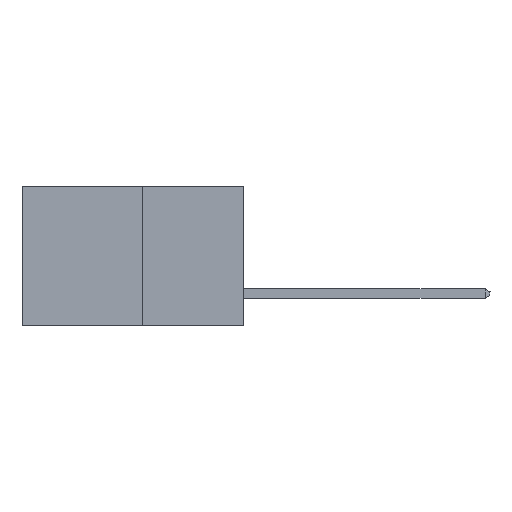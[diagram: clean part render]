
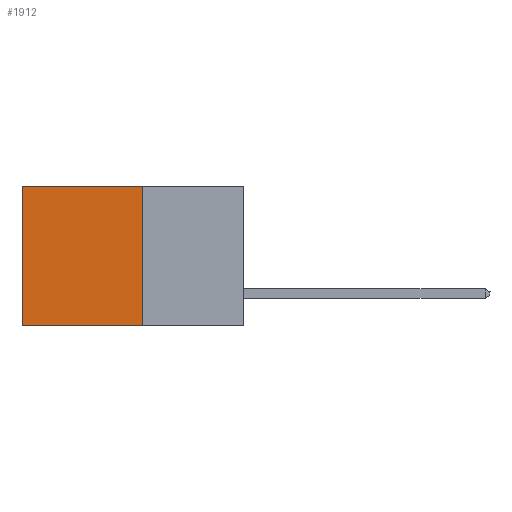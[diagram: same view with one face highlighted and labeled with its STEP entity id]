
A CAD part, left-side view. The second image highlights one B-rep face of the part: STEP entity #1912.
In plain terms, the highlighted planar face has unit normal (-1, 0, 0).
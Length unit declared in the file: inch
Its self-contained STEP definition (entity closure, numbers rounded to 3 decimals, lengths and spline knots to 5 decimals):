
#285 = EDGE_CURVE ( 'NONE', #6637, #10688, #9355, .T. ) ;
#1652 = CARTESIAN_POINT ( 'NONE',  ( 0.277, 0.27, -0.37 ) ) ;
#1794 = DIRECTION ( 'NONE',  ( 0., 0., -1. ) ) ;
#1912 = ADVANCED_FACE ( 'NONE', ( #9507 ), #6419, .F. ) ;
#2110 = CARTESIAN_POINT ( 'NONE',  ( 0.277, 0.27, -0.37 ) ) ;
#2352 = CARTESIAN_POINT ( 'NONE',  ( 0.277, 0.59, -0.37 ) ) ;
#2558 = DIRECTION ( 'NONE',  ( 0., 0., -1. ) ) ;
#3580 = ORIENTED_EDGE ( 'NONE', *, *, #6530, .T. ) ;
#3706 = CARTESIAN_POINT ( 'NONE',  ( 0.277, 0.27, 0. ) ) ;
#3796 = ORIENTED_EDGE ( 'NONE', *, *, #285, .F. ) ;
#3920 = ORIENTED_EDGE ( 'NONE', *, *, #5425, .F. ) ;
#4307 = ORIENTED_EDGE ( 'NONE', *, *, #9926, .T. ) ;
#4753 = DIRECTION ( 'NONE',  ( 0., 1., 0. ) ) ;
#5056 = AXIS2_PLACEMENT_3D ( 'NONE', #6396, #5975, #5937 ) ;
#5283 = VECTOR ( 'NONE', #4753, 39.37008 ) ;
#5425 = EDGE_CURVE ( 'NONE', #9113, #6637, #10570, .T. ) ;
#5875 = CARTESIAN_POINT ( 'NONE',  ( 0.277, 0.27, -0.37 ) ) ;
#5937 = DIRECTION ( 'NONE',  ( 0., 0., -1. ) ) ;
#5975 = DIRECTION ( 'NONE',  ( 1., 0., 0. ) ) ;
#6396 = CARTESIAN_POINT ( 'NONE',  ( 0.277, 0.27, -0.37 ) ) ;
#6419 = PLANE ( 'NONE',  #5056 ) ;
#6530 = EDGE_CURVE ( 'NONE', #11712, #10688, #10371, .T. ) ;
#6637 = VERTEX_POINT ( 'NONE', #1652 ) ;
#6646 = VECTOR ( 'NONE', #9625, 39.37008 ) ;
#7400 = CARTESIAN_POINT ( 'NONE',  ( 0.277, 0.27, 0. ) ) ;
#8408 = LINE ( 'NONE', #3706, #5283 ) ;
#9113 = VERTEX_POINT ( 'NONE', #7400 ) ;
#9355 = LINE ( 'NONE', #5875, #6646 ) ;
#9507 = FACE_OUTER_BOUND ( 'NONE', #9628, .T. ) ;
#9625 = DIRECTION ( 'NONE',  ( 0., 1., 0. ) ) ;
#9628 = EDGE_LOOP ( 'NONE', ( #3580, #3796, #3920, #4307 ) ) ;
#9806 = CARTESIAN_POINT ( 'NONE',  ( 0.277, 0.59, -0.37 ) ) ;
#9926 = EDGE_CURVE ( 'NONE', #9113, #11712, #8408, .T. ) ;
#10077 = VECTOR ( 'NONE', #2558, 39.37008 ) ;
#10371 = LINE ( 'NONE', #9806, #10077 ) ;
#10570 = LINE ( 'NONE', #2110, #12248 ) ;
#10688 = VERTEX_POINT ( 'NONE', #2352 ) ;
#11712 = VERTEX_POINT ( 'NONE', #12154 ) ;
#12154 = CARTESIAN_POINT ( 'NONE',  ( 0.277, 0.59, 0. ) ) ;
#12248 = VECTOR ( 'NONE', #1794, 39.37008 ) ;
